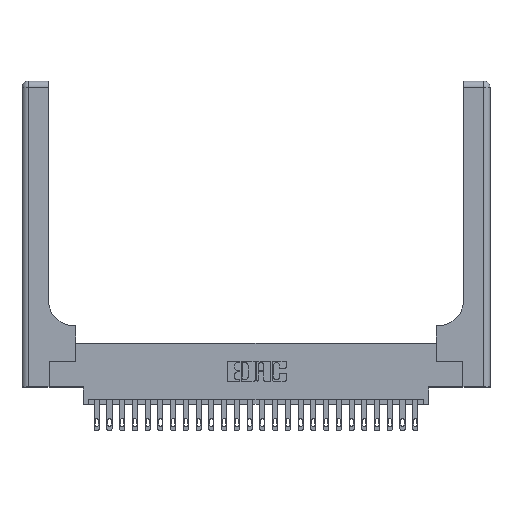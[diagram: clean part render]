
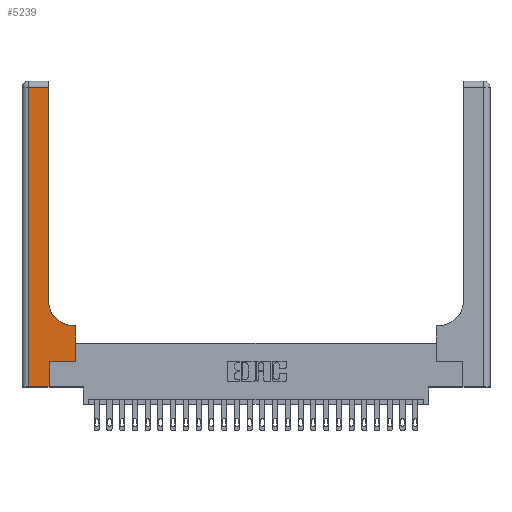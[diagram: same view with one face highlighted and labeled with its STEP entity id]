
A CAD part, top view. The second image highlights one B-rep face of the part: STEP entity #5239.
In plain terms, the highlighted planar face has unit normal (0, 0, 1).
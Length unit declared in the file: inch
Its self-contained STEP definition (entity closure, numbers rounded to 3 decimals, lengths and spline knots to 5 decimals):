
#581 = ORIENTED_EDGE ( 'NONE', *, *, #8868, .T. ) ;
#609 = ORIENTED_EDGE ( 'NONE', *, *, #18498, .T. ) ;
#617 = VECTOR ( 'NONE', #20144, 39.37008 ) ;
#1087 = PLANE ( 'NONE',  #10458 ) ;
#1500 = CARTESIAN_POINT ( 'NONE',  ( 0.26, 2.94, 0.37 ) ) ;
#1662 = CARTESIAN_POINT ( 'NONE',  ( 0.51, 0.6, 0.37 ) ) ;
#1818 = CARTESIAN_POINT ( 'NONE',  ( 0.528, 0.25, 0.37 ) ) ;
#1837 = CARTESIAN_POINT ( 'NONE',  ( 0.265, 0., 0.37 ) ) ;
#1922 = DIRECTION ( 'NONE',  ( -1., 0., 0. ) ) ;
#2391 = EDGE_CURVE ( 'NONE', #24049, #15700, #16513, .T. ) ;
#2512 = EDGE_CURVE ( 'NONE', #19898, #11419, #22558, .T. ) ;
#2672 = CARTESIAN_POINT ( 'NONE',  ( 0.06, 0., 0.37 ) ) ;
#2750 = DIRECTION ( 'NONE',  ( 0., 0., -1. ) ) ;
#3055 = LINE ( 'NONE', #10010, #9142 ) ;
#3439 = LINE ( 'NONE', #3550, #6285 ) ;
#3550 = CARTESIAN_POINT ( 'NONE',  ( 0.06, 3., 0.37 ) ) ;
#4486 = FACE_OUTER_BOUND ( 'NONE', #17316, .T. ) ;
#4612 = CARTESIAN_POINT ( 'NONE',  ( 0., 0., 0.37 ) ) ;
#4730 = CARTESIAN_POINT ( 'NONE',  ( 0., 2.94, 0.37 ) ) ;
#5166 = CARTESIAN_POINT ( 'NONE',  ( 0.06, 2.94, 0.37 ) ) ;
#5239 = ADVANCED_FACE ( 'NONE', ( #4486 ), #1087, .F. ) ;
#5384 = CIRCLE ( 'NONE', #6998, 0.25 ) ;
#5648 = CARTESIAN_POINT ( 'NONE',  ( 0.528, 0.6, 0.37 ) ) ;
#6027 = LINE ( 'NONE', #21223, #13978 ) ;
#6106 = CARTESIAN_POINT ( 'NONE',  ( 0.26, 3., 0.37 ) ) ;
#6136 = DIRECTION ( 'NONE',  ( 1., 0., 0. ) ) ;
#6285 = VECTOR ( 'NONE', #22534, 39.37008 ) ;
#6299 = VECTOR ( 'NONE', #20033, 39.37008 ) ;
#6374 = DIRECTION ( 'NONE',  ( -1., 0., 0. ) ) ;
#6620 = DIRECTION ( 'NONE',  ( 0., 0., -1. ) ) ;
#6808 = CARTESIAN_POINT ( 'NONE',  ( 0.265, 0.25, 0.37 ) ) ;
#6998 = AXIS2_PLACEMENT_3D ( 'NONE', #21846, #2750, #6136 ) ;
#7213 = EDGE_CURVE ( 'NONE', #11419, #22280, #5384, .T. ) ;
#7750 = ORIENTED_EDGE ( 'NONE', *, *, #13114, .T. ) ;
#7756 = LINE ( 'NONE', #1837, #18710 ) ;
#8868 = EDGE_CURVE ( 'NONE', #24728, #22179, #7756, .T. ) ;
#8875 = ORIENTED_EDGE ( 'NONE', *, *, #18009, .T. ) ;
#9129 = VECTOR ( 'NONE', #14026, 39.37008 ) ;
#9142 = VECTOR ( 'NONE', #17627, 39.37008 ) ;
#9389 = ORIENTED_EDGE ( 'NONE', *, *, #7213, .T. ) ;
#9862 = VECTOR ( 'NONE', #1922, 39.37008 ) ;
#9985 = CARTESIAN_POINT ( 'NONE',  ( 0.26, 0.85, 0.37 ) ) ;
#10010 = CARTESIAN_POINT ( 'NONE',  ( 0.265, 0.25, 0.37 ) ) ;
#10458 = AXIS2_PLACEMENT_3D ( 'NONE', #12663, #6620, #6374 ) ;
#10774 = LINE ( 'NONE', #4612, #6299 ) ;
#11419 = VERTEX_POINT ( 'NONE', #1662 ) ;
#11495 = CARTESIAN_POINT ( 'NONE',  ( 0.265, 0., 0.37 ) ) ;
#12020 = ORIENTED_EDGE ( 'NONE', *, *, #19869, .T. ) ;
#12663 = CARTESIAN_POINT ( 'NONE',  ( 0., 3., 0.37 ) ) ;
#13114 = EDGE_CURVE ( 'NONE', #22179, #17893, #3055, .T. ) ;
#13497 = CARTESIAN_POINT ( 'NONE',  ( 0.26, 0.6, 0.37 ) ) ;
#13691 = DIRECTION ( 'NONE',  ( 0., 1., 0. ) ) ;
#13978 = VECTOR ( 'NONE', #13691, 39.37008 ) ;
#14026 = DIRECTION ( 'NONE',  ( 0., 1., 0. ) ) ;
#15283 = ORIENTED_EDGE ( 'NONE', *, *, #18679, .T. ) ;
#15700 = VERTEX_POINT ( 'NONE', #5166 ) ;
#16214 = ORIENTED_EDGE ( 'NONE', *, *, #2512, .T. ) ;
#16513 = LINE ( 'NONE', #4730, #617 ) ;
#17316 = EDGE_LOOP ( 'NONE', ( #609, #20868, #8875, #15283, #581, #7750, #12020, #16214, #9389 ) ) ;
#17401 = LINE ( 'NONE', #6106, #9129 ) ;
#17627 = DIRECTION ( 'NONE',  ( 1., 0., 0. ) ) ;
#17893 = VERTEX_POINT ( 'NONE', #1818 ) ;
#18009 = EDGE_CURVE ( 'NONE', #15700, #22410, #3439, .T. ) ;
#18498 = EDGE_CURVE ( 'NONE', #22280, #24049, #17401, .T. ) ;
#18679 = EDGE_CURVE ( 'NONE', #22410, #24728, #10774, .T. ) ;
#18710 = VECTOR ( 'NONE', #24601, 39.37008 ) ;
#19869 = EDGE_CURVE ( 'NONE', #17893, #19898, #6027, .T. ) ;
#19898 = VERTEX_POINT ( 'NONE', #5648 ) ;
#20033 = DIRECTION ( 'NONE',  ( 1., 0., 0. ) ) ;
#20144 = DIRECTION ( 'NONE',  ( -1., 0., 0. ) ) ;
#20868 = ORIENTED_EDGE ( 'NONE', *, *, #2391, .T. ) ;
#21223 = CARTESIAN_POINT ( 'NONE',  ( 0.528, 0.25, 0.37 ) ) ;
#21846 = CARTESIAN_POINT ( 'NONE',  ( 0.51, 0.85, 0.37 ) ) ;
#22179 = VERTEX_POINT ( 'NONE', #6808 ) ;
#22280 = VERTEX_POINT ( 'NONE', #9985 ) ;
#22410 = VERTEX_POINT ( 'NONE', #2672 ) ;
#22534 = DIRECTION ( 'NONE',  ( 0., -1., 0. ) ) ;
#22558 = LINE ( 'NONE', #13497, #9862 ) ;
#24049 = VERTEX_POINT ( 'NONE', #1500 ) ;
#24601 = DIRECTION ( 'NONE',  ( 0., 1., 0. ) ) ;
#24728 = VERTEX_POINT ( 'NONE', #11495 ) ;
